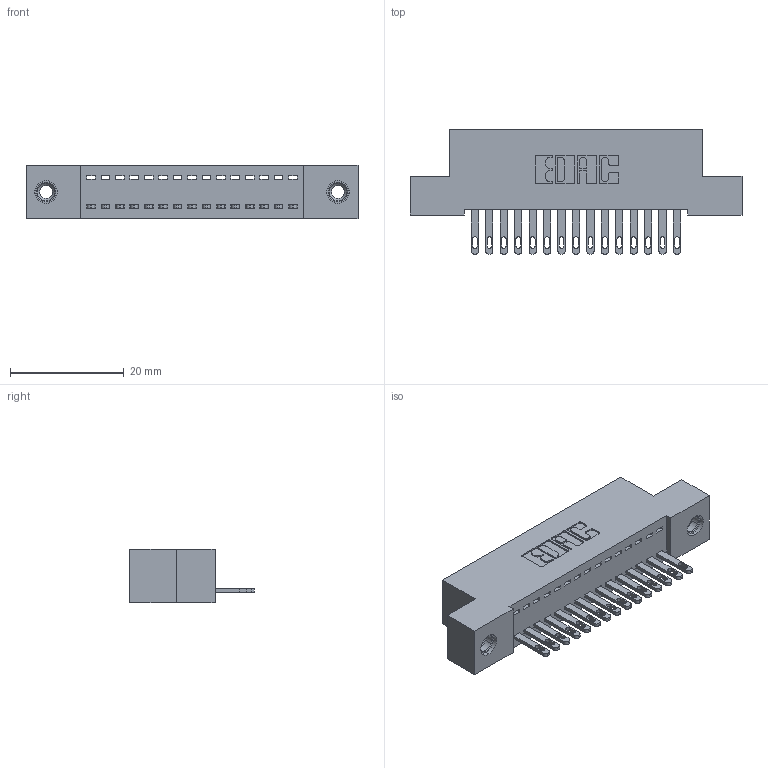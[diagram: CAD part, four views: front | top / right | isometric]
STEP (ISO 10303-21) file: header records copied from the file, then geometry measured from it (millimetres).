
FILE_DESCRIPTION (( 'STEP AP203' ), '1' );
FILE_NAME ('892-015-500-108.STEP', '2020-09-21T13:23:07', ( '' ), ( '' ), 'SwSTEP 2.0', 'SolidWorks 2020', '' );
FILE_SCHEMA (( 'CONFIG_CONTROL_DESIGN' ));
Length unit declared in the file: inch
Products named in the file (4): 345-292-001_345-293-100; 842 Part_TI; 892-015-500-108; 345-250-001_345-250-003-102
Assembly tree (18 placements, depth 2):
  892-015-500-108
    842 Part_TI
    345-292-001_345-293-100  x15
    345-250-001_345-250-003-102  x2
Bounding box: 58.42 x 21.85 x 9.4 mm (x, y, z)
Volume: 5026.4 mm3; surface area: 6924.3 mm2
Topology: 18 solids, 18 shells, 980 faces, 2955 edges, 1962 vertices
Faces by surface type: plane 638, cylinder 326, cone 12, torus 4
Entity records: 13646 total; most frequent: CARTESIAN_POINT 2338, ORIENTED_EDGE 2282, DIRECTION 2061, EDGE_CURVE 1141, VECTOR 989, LINE 989, VERTEX_POINT 756, AXIS2_PLACEMENT_3D 536
